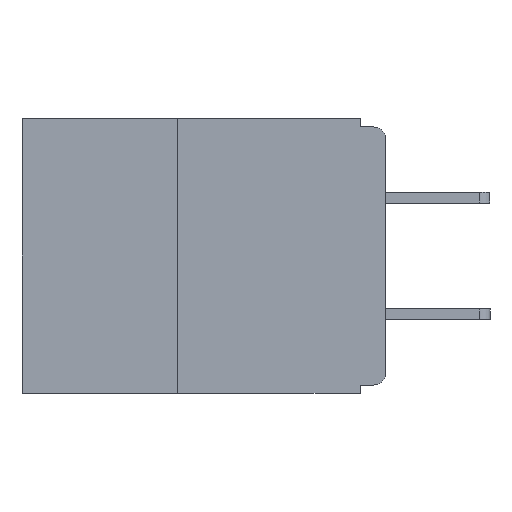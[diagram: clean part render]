
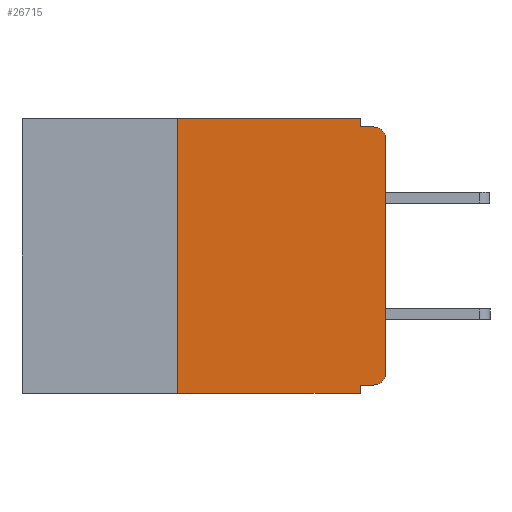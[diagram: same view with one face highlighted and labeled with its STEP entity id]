
A CAD part, left-side view. The second image highlights one B-rep face of the part: STEP entity #26715.
In plain terms, the highlighted planar face has unit normal (-1, 0, 0).
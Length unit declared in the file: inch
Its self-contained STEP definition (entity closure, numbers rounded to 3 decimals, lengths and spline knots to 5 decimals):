
#421 = ORIENTED_EDGE ( 'NONE', *, *, #21141, .T. ) ;
#980 = DIRECTION ( 'NONE',  ( 0., 0., -1. ) ) ;
#1217 = DIRECTION ( 'NONE',  ( 0., -1., 0. ) ) ;
#1335 = DIRECTION ( 'NONE',  ( 0., 0., -1. ) ) ;
#1537 = CIRCLE ( 'NONE', #21139, 0.015 ) ;
#1992 = LINE ( 'NONE', #14195, #25486 ) ;
#2398 = VECTOR ( 'NONE', #26843, 39.37008 ) ;
#2620 = CARTESIAN_POINT ( 'NONE',  ( 0., 0.015, -0.01 ) ) ;
#2692 = VECTOR ( 'NONE', #8534, 39.37008 ) ;
#2852 = CARTESIAN_POINT ( 'NONE',  ( 0., 0.437, 0. ) ) ;
#3195 = VERTEX_POINT ( 'NONE', #14455 ) ;
#3257 = VERTEX_POINT ( 'NONE', #16914 ) ;
#3808 = EDGE_CURVE ( 'NONE', #5632, #27350, #4623, .T. ) ;
#4038 = DIRECTION ( 'NONE',  ( 0., 0., 1. ) ) ;
#4242 = LINE ( 'NONE', #14961, #22489 ) ;
#4382 = EDGE_CURVE ( 'NONE', #23594, #21558, #1992, .T. ) ;
#4623 = LINE ( 'NONE', #17725, #28004 ) ;
#5632 = VERTEX_POINT ( 'NONE', #12162 ) ;
#5724 = VERTEX_POINT ( 'NONE', #14736 ) ;
#6457 = ORIENTED_EDGE ( 'NONE', *, *, #18804, .F. ) ;
#6498 = ORIENTED_EDGE ( 'NONE', *, *, #13998, .F. ) ;
#7512 = EDGE_CURVE ( 'NONE', #22034, #5632, #10826, .T. ) ;
#7525 = PLANE ( 'NONE',  #14939 ) ;
#8534 = DIRECTION ( 'NONE',  ( 0., 0., 1. ) ) ;
#8590 = CARTESIAN_POINT ( 'NONE',  ( 0., 0.031, -0.33 ) ) ;
#9347 = EDGE_LOOP ( 'NONE', ( #22742, #421, #20326, #22098, #12064, #15279, #11333, #6457, #6498, #10442 ) ) ;
#9747 = DIRECTION ( 'NONE',  ( 0., -1., 0. ) ) ;
#9838 = DIRECTION ( 'NONE',  ( 0., 0., -1. ) ) ;
#10051 = EDGE_CURVE ( 'NONE', #5724, #25854, #16038, .T. ) ;
#10442 = ORIENTED_EDGE ( 'NONE', *, *, #7512, .T. ) ;
#10826 = CIRCLE ( 'NONE', #16289, 0.015 ) ;
#10831 = CARTESIAN_POINT ( 'NONE',  ( 0., 0.437, -0.33 ) ) ;
#11333 = ORIENTED_EDGE ( 'NONE', *, *, #10051, .T. ) ;
#11547 = EDGE_CURVE ( 'NONE', #5724, #17351, #27553, .T. ) ;
#12064 = ORIENTED_EDGE ( 'NONE', *, *, #18092, .F. ) ;
#12162 = CARTESIAN_POINT ( 'NONE',  ( 0., 0., -0.305 ) ) ;
#13091 = DIRECTION ( 'NONE',  ( 0., -1., 0. ) ) ;
#13235 = DIRECTION ( 'NONE',  ( 0., 1., 0. ) ) ;
#13998 = EDGE_CURVE ( 'NONE', #22034, #3195, #24985, .T. ) ;
#14195 = CARTESIAN_POINT ( 'NONE',  ( 0., 0., -0.01 ) ) ;
#14455 = CARTESIAN_POINT ( 'NONE',  ( 0., 0.031, -0.32 ) ) ;
#14539 = CARTESIAN_POINT ( 'NONE',  ( 0., 0., -0.025 ) ) ;
#14736 = CARTESIAN_POINT ( 'NONE',  ( 0., 0.25, -0.33 ) ) ;
#14742 = DIRECTION ( 'NONE',  ( -1., 0., 0. ) ) ;
#14939 = AXIS2_PLACEMENT_3D ( 'NONE', #2852, #23412, #9838 ) ;
#14961 = CARTESIAN_POINT ( 'NONE',  ( 0., 0.437, 0. ) ) ;
#15072 = DIRECTION ( 'NONE',  ( -1., 0., 0. ) ) ;
#15279 = ORIENTED_EDGE ( 'NONE', *, *, #11547, .F. ) ;
#15314 = VECTOR ( 'NONE', #13091, 39.37008 ) ;
#16038 = LINE ( 'NONE', #10831, #15314 ) ;
#16289 = AXIS2_PLACEMENT_3D ( 'NONE', #28177, #14742, #980 ) ;
#16907 = VECTOR ( 'NONE', #20173, 39.37008 ) ;
#16914 = CARTESIAN_POINT ( 'NONE',  ( 0., 0.031, 0. ) ) ;
#17351 = VERTEX_POINT ( 'NONE', #19044 ) ;
#17638 = CARTESIAN_POINT ( 'NONE',  ( 0., 0.25, -0.33 ) ) ;
#17725 = CARTESIAN_POINT ( 'NONE',  ( 0., 0., 0. ) ) ;
#18092 = EDGE_CURVE ( 'NONE', #17351, #3257, #4242, .T. ) ;
#18804 = EDGE_CURVE ( 'NONE', #3195, #25854, #20646, .T. ) ;
#18969 = VECTOR ( 'NONE', #13235, 39.37008 ) ;
#19044 = CARTESIAN_POINT ( 'NONE',  ( 0., 0.25, 0. ) ) ;
#20173 = DIRECTION ( 'NONE',  ( 0., 0., -1. ) ) ;
#20326 = ORIENTED_EDGE ( 'NONE', *, *, #4382, .F. ) ;
#20646 = LINE ( 'NONE', #24633, #2398 ) ;
#21139 = AXIS2_PLACEMENT_3D ( 'NONE', #28496, #15072, #1335 ) ;
#21141 = EDGE_CURVE ( 'NONE', #27350, #21558, #1537, .T. ) ;
#21558 = VERTEX_POINT ( 'NONE', #2620 ) ;
#22034 = VERTEX_POINT ( 'NONE', #27041 ) ;
#22098 = ORIENTED_EDGE ( 'NONE', *, *, #26438, .F. ) ;
#22489 = VECTOR ( 'NONE', #1217, 39.37008 ) ;
#22742 = ORIENTED_EDGE ( 'NONE', *, *, #3808, .T. ) ;
#23412 = DIRECTION ( 'NONE',  ( 1., 0., 0. ) ) ;
#23594 = VERTEX_POINT ( 'NONE', #25595 ) ;
#24633 = CARTESIAN_POINT ( 'NONE',  ( 0., 0.031, -0.33 ) ) ;
#24985 = LINE ( 'NONE', #28917, #18969 ) ;
#25486 = VECTOR ( 'NONE', #9747, 39.37008 ) ;
#25595 = CARTESIAN_POINT ( 'NONE',  ( 0., 0.031, -0.01 ) ) ;
#25854 = VERTEX_POINT ( 'NONE', #8590 ) ;
#26409 = FACE_OUTER_BOUND ( 'NONE', #9347, .T. ) ;
#26438 = EDGE_CURVE ( 'NONE', #3257, #23594, #28824, .T. ) ;
#26715 = ADVANCED_FACE ( 'NONE', ( #26409 ), #7525, .F. ) ;
#26843 = DIRECTION ( 'NONE',  ( 0., 0., -1. ) ) ;
#27041 = CARTESIAN_POINT ( 'NONE',  ( 0., 0.015, -0.32 ) ) ;
#27350 = VERTEX_POINT ( 'NONE', #14539 ) ;
#27553 = LINE ( 'NONE', #17638, #2692 ) ;
#28004 = VECTOR ( 'NONE', #4038, 39.37008 ) ;
#28177 = CARTESIAN_POINT ( 'NONE',  ( 0., 0.015, -0.305 ) ) ;
#28496 = CARTESIAN_POINT ( 'NONE',  ( 0., 0.015, -0.025 ) ) ;
#28824 = LINE ( 'NONE', #29006, #16907 ) ;
#28917 = CARTESIAN_POINT ( 'NONE',  ( 0., 0., -0.32 ) ) ;
#29006 = CARTESIAN_POINT ( 'NONE',  ( 0., 0.031, 0. ) ) ;
